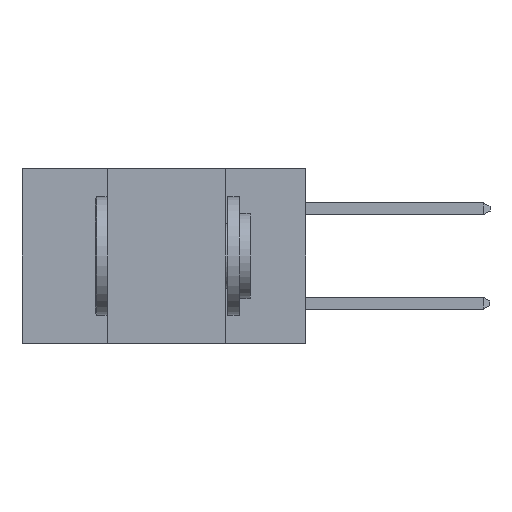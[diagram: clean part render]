
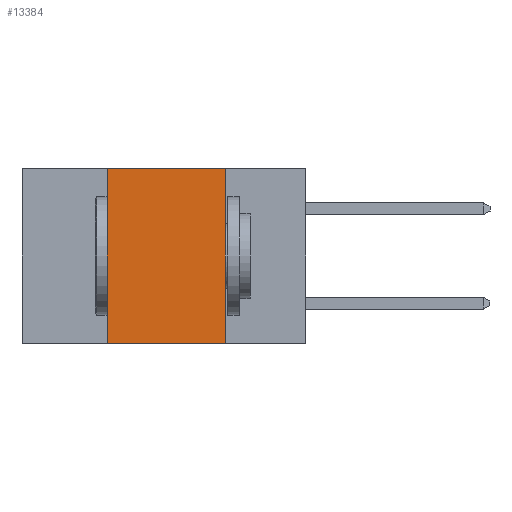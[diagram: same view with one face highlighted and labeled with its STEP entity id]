
A CAD part, left-side view. The second image highlights one B-rep face of the part: STEP entity #13384.
In plain terms, the highlighted planar face has unit normal (-1, 0, 0).
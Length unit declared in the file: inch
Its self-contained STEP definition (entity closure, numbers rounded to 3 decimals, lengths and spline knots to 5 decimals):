
#559 = DIRECTION ( 'NONE',  ( 0., -1., 0. ) ) ;
#629 = CARTESIAN_POINT ( 'NONE',  ( 0., 0.6, -0.37 ) ) ;
#640 = LINE ( 'NONE', #629, #11265 ) ;
#2051 = VERTEX_POINT ( 'NONE', #13077 ) ;
#2063 = DIRECTION ( 'NONE',  ( 0., -1., 0. ) ) ;
#2449 = CARTESIAN_POINT ( 'NONE',  ( 0., 0.17, 0. ) ) ;
#2472 = AXIS2_PLACEMENT_3D ( 'NONE', #5625, #7011, #16583 ) ;
#2642 = ORIENTED_EDGE ( 'NONE', *, *, #15734, .F. ) ;
#2756 = VECTOR ( 'NONE', #559, 39.37008 ) ;
#2816 = FACE_OUTER_BOUND ( 'NONE', #4152, .T. ) ;
#2967 = VERTEX_POINT ( 'NONE', #15475 ) ;
#3936 = DIRECTION ( 'NONE',  ( 0., 0., -1. ) ) ;
#4152 = EDGE_LOOP ( 'NONE', ( #15873, #2642, #11568, #11225 ) ) ;
#4290 = VECTOR ( 'NONE', #11424, 39.37008 ) ;
#5008 = VECTOR ( 'NONE', #3936, 39.37008 ) ;
#5625 = CARTESIAN_POINT ( 'NONE',  ( 0., 0.6, 0. ) ) ;
#5657 = VERTEX_POINT ( 'NONE', #6540 ) ;
#6540 = CARTESIAN_POINT ( 'NONE',  ( 0., 0.17, 0. ) ) ;
#7011 = DIRECTION ( 'NONE',  ( 1., 0., 0. ) ) ;
#10050 = CARTESIAN_POINT ( 'NONE',  ( 0., 0.42, 0. ) ) ;
#10067 = LINE ( 'NONE', #15739, #2756 ) ;
#11225 = ORIENTED_EDGE ( 'NONE', *, *, #11738, .T. ) ;
#11265 = VECTOR ( 'NONE', #2063, 39.37008 ) ;
#11424 = DIRECTION ( 'NONE',  ( 0., 0., 1. ) ) ;
#11568 = ORIENTED_EDGE ( 'NONE', *, *, #14969, .F. ) ;
#11577 = LINE ( 'NONE', #10050, #4290 ) ;
#11738 = EDGE_CURVE ( 'NONE', #2967, #2051, #640, .T. ) ;
#12384 = VERTEX_POINT ( 'NONE', #15900 ) ;
#13077 = CARTESIAN_POINT ( 'NONE',  ( 0., 0.17, -0.37 ) ) ;
#13235 = EDGE_CURVE ( 'NONE', #5657, #2051, #16789, .T. ) ;
#13384 = ADVANCED_FACE ( 'NONE', ( #2816 ), #13816, .F. ) ;
#13816 = PLANE ( 'NONE',  #2472 ) ;
#14969 = EDGE_CURVE ( 'NONE', #2967, #12384, #11577, .T. ) ;
#15475 = CARTESIAN_POINT ( 'NONE',  ( 0., 0.42, -0.37 ) ) ;
#15734 = EDGE_CURVE ( 'NONE', #12384, #5657, #10067, .T. ) ;
#15739 = CARTESIAN_POINT ( 'NONE',  ( 0., 0.6, 0. ) ) ;
#15873 = ORIENTED_EDGE ( 'NONE', *, *, #13235, .F. ) ;
#15900 = CARTESIAN_POINT ( 'NONE',  ( 0., 0.42, 0. ) ) ;
#16583 = DIRECTION ( 'NONE',  ( 0., 0., -1. ) ) ;
#16789 = LINE ( 'NONE', #2449, #5008 ) ;
